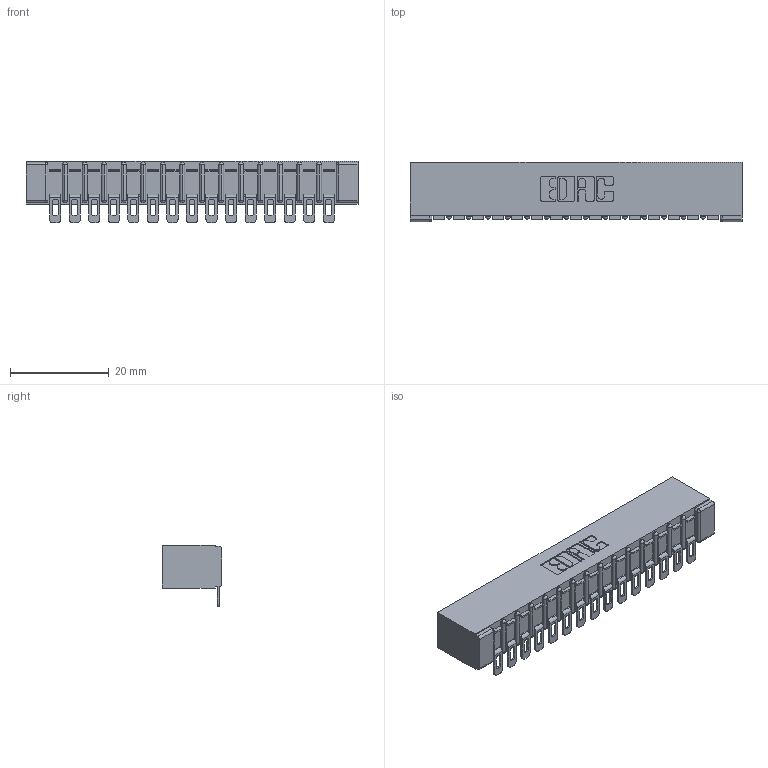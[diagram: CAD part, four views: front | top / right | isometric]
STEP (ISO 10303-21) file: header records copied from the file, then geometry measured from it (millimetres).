
FILE_DESCRIPTION (( 'STEP AP203' ), '1' );
FILE_NAME ('307-015-554-101.STEP', '2019-09-04T21:04:59', ( '' ), ( '' ), 'SwSTEP 2.0', 'SolidWorks 2016', '' );
FILE_SCHEMA (( 'CONFIG_CONTROL_DESIGN' ));
Length unit declared in the file: inch
Products named in the file (3): 307-015-554-101; 307 Part_No Mounting Lugs; 307-290-002_554
Assembly tree (16 placements, depth 2):
  307-015-554-101
    307 Part_No Mounting Lugs
    307-290-002_554  x15
Bounding box: 67.31 x 12.01 x 12.52 mm (x, y, z)
Volume: 4687.7 mm3; surface area: 8705.9 mm2
Topology: 16 solids, 16 shells, 1341 faces, 4094 edges, 2684 vertices
Faces by surface type: plane 756, cylinder 553, sphere 32
Entity records: 16875 total; most frequent: CARTESIAN_POINT 2842, ORIENTED_EDGE 2832, DIRECTION 2778, EDGE_CURVE 1416, VECTOR 1066, LINE 1066, VERTEX_POINT 920, AXIS2_PLACEMENT_3D 856
